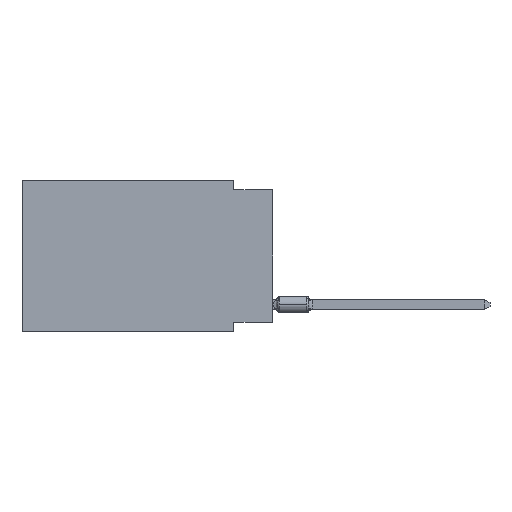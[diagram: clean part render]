
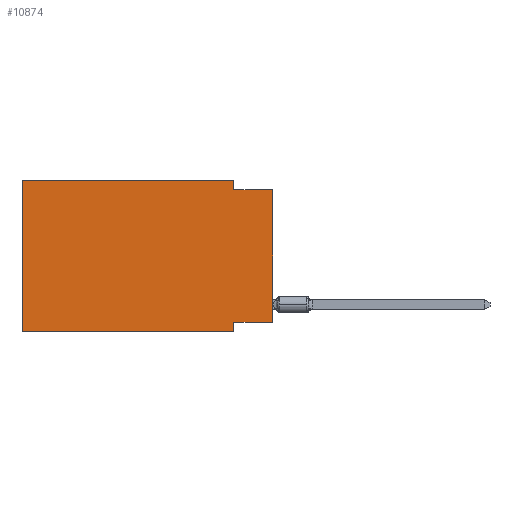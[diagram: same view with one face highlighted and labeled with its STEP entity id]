
A CAD part, left-side view. The second image highlights one B-rep face of the part: STEP entity #10874.
In plain terms, the highlighted planar face has unit normal (-1, 0, 0).
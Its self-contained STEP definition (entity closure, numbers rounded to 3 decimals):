
#380 = VERTEX_POINT ( 'NONE', #16516 ) ;
#742 = EDGE_CURVE ( 'NONE', #9651, #5058, #17150, .T. ) ;
#1003 = DIRECTION ( 'NONE',  ( 0., 0., -1. ) ) ;
#1548 = CARTESIAN_POINT ( 'NONE',  ( 0., 0., -0.635 ) ) ;
#1656 = ORIENTED_EDGE ( 'NONE', *, *, #742, .F. ) ;
#2826 = LINE ( 'NONE', #12935, #8283 ) ;
#3084 = LINE ( 'NONE', #5851, #5185 ) ;
#3641 = EDGE_CURVE ( 'NONE', #5058, #5404, #4393, .T. ) ;
#3716 = ORIENTED_EDGE ( 'NONE', *, *, #12980, .F. ) ;
#3923 = VECTOR ( 'NONE', #11103, 1000. ) ;
#4070 = AXIS2_PLACEMENT_3D ( 'NONE', #16251, #11165, #17633 ) ;
#4078 = DIRECTION ( 'NONE',  ( 0., 1., 0. ) ) ;
#4393 = LINE ( 'NONE', #10900, #8874 ) ;
#5058 = VERTEX_POINT ( 'NONE', #15827 ) ;
#5185 = VECTOR ( 'NONE', #14366, 1000. ) ;
#5404 = VERTEX_POINT ( 'NONE', #14855 ) ;
#5851 = CARTESIAN_POINT ( 'NONE',  ( 0., 16.383, -9.906 ) ) ;
#6020 = VECTOR ( 'NONE', #6716, 1000. ) ;
#6108 = DIRECTION ( 'NONE',  ( 0., 0., -1. ) ) ;
#6399 = VECTOR ( 'NONE', #20626, 1000. ) ;
#6577 = CARTESIAN_POINT ( 'NONE',  ( 0., 16.383, 0. ) ) ;
#6716 = DIRECTION ( 'NONE',  ( 0., -1., 0. ) ) ;
#7684 = CARTESIAN_POINT ( 'NONE',  ( 0., 16.383, -9.906 ) ) ;
#7973 = FACE_OUTER_BOUND ( 'NONE', #18762, .T. ) ;
#7992 = CARTESIAN_POINT ( 'NONE',  ( 0., 0., -9.271 ) ) ;
#8283 = VECTOR ( 'NONE', #6108, 1000. ) ;
#8499 = ORIENTED_EDGE ( 'NONE', *, *, #3641, .F. ) ;
#8543 = ORIENTED_EDGE ( 'NONE', *, *, #11655, .F. ) ;
#8678 = VERTEX_POINT ( 'NONE', #6577 ) ;
#8874 = VECTOR ( 'NONE', #1003, 1000. ) ;
#9651 = VERTEX_POINT ( 'NONE', #13818 ) ;
#9938 = ORIENTED_EDGE ( 'NONE', *, *, #14705, .T. ) ;
#10072 = ORIENTED_EDGE ( 'NONE', *, *, #20244, .F. ) ;
#10818 = VECTOR ( 'NONE', #4078, 1000. ) ;
#10874 = ADVANCED_FACE ( 'NONE', ( #7973 ), #11061, .F. ) ;
#10900 = CARTESIAN_POINT ( 'NONE',  ( 0., 2.54, -9.906 ) ) ;
#11061 = PLANE ( 'NONE',  #4070 ) ;
#11103 = DIRECTION ( 'NONE',  ( 0., -1., 0. ) ) ;
#11165 = DIRECTION ( 'NONE',  ( 1., 0., 0. ) ) ;
#11655 = EDGE_CURVE ( 'NONE', #13703, #20889, #16101, .T. ) ;
#12462 = CARTESIAN_POINT ( 'NONE',  ( 0., 16.383, 0. ) ) ;
#12913 = CARTESIAN_POINT ( 'NONE',  ( 0., 16.383, 0. ) ) ;
#12935 = CARTESIAN_POINT ( 'NONE',  ( 0., 2.54, 0. ) ) ;
#12980 = EDGE_CURVE ( 'NONE', #20616, #8678, #20742, .T. ) ;
#13703 = VERTEX_POINT ( 'NONE', #16458 ) ;
#13818 = CARTESIAN_POINT ( 'NONE',  ( 0., 0., -9.271 ) ) ;
#13899 = DIRECTION ( 'NONE',  ( 0., 0., 1. ) ) ;
#14366 = DIRECTION ( 'NONE',  ( 0., -1., 0. ) ) ;
#14705 = EDGE_CURVE ( 'NONE', #20616, #5404, #3084, .T. ) ;
#14855 = CARTESIAN_POINT ( 'NONE',  ( 0., 2.54, -9.906 ) ) ;
#15762 = EDGE_CURVE ( 'NONE', #9651, #20889, #17296, .T. ) ;
#15827 = CARTESIAN_POINT ( 'NONE',  ( 0., 2.54, -9.271 ) ) ;
#16101 = LINE ( 'NONE', #1548, #6020 ) ;
#16129 = ORIENTED_EDGE ( 'NONE', *, *, #15762, .T. ) ;
#16251 = CARTESIAN_POINT ( 'NONE',  ( 0., 16.383, 0. ) ) ;
#16448 = ORIENTED_EDGE ( 'NONE', *, *, #20652, .F. ) ;
#16458 = CARTESIAN_POINT ( 'NONE',  ( 0., 2.54, -0.635 ) ) ;
#16516 = CARTESIAN_POINT ( 'NONE',  ( 0., 2.54, 0. ) ) ;
#16787 = VECTOR ( 'NONE', #13899, 1000. ) ;
#17150 = LINE ( 'NONE', #7992, #10818 ) ;
#17296 = LINE ( 'NONE', #20379, #16787 ) ;
#17307 = CARTESIAN_POINT ( 'NONE',  ( 0., 0., -0.635 ) ) ;
#17633 = DIRECTION ( 'NONE',  ( 0., 0., -1. ) ) ;
#18762 = EDGE_LOOP ( 'NONE', ( #16129, #8543, #10072, #16448, #3716, #9938, #8499, #1656 ) ) ;
#18967 = LINE ( 'NONE', #12913, #3923 ) ;
#20244 = EDGE_CURVE ( 'NONE', #380, #13703, #2826, .T. ) ;
#20379 = CARTESIAN_POINT ( 'NONE',  ( 0., 0., 0. ) ) ;
#20616 = VERTEX_POINT ( 'NONE', #7684 ) ;
#20626 = DIRECTION ( 'NONE',  ( 0., 0., 1. ) ) ;
#20652 = EDGE_CURVE ( 'NONE', #8678, #380, #18967, .T. ) ;
#20742 = LINE ( 'NONE', #12462, #6399 ) ;
#20889 = VERTEX_POINT ( 'NONE', #17307 ) ;
